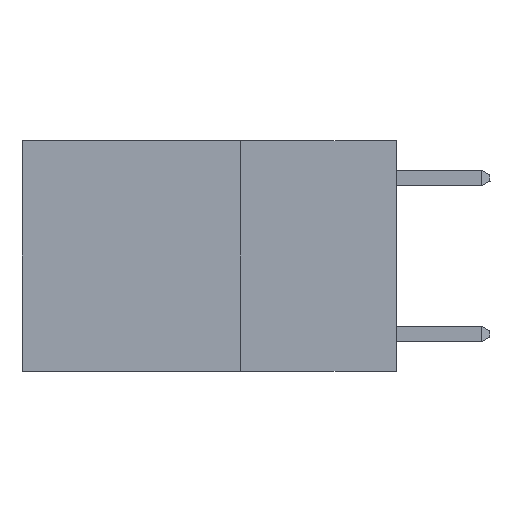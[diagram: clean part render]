
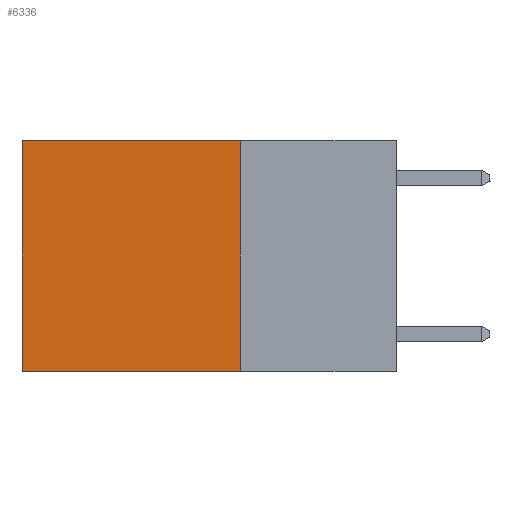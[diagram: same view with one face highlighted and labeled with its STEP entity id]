
A CAD part, left-side view. The second image highlights one B-rep face of the part: STEP entity #6336.
In plain terms, the highlighted planar face has unit normal (-1, 0, 0).
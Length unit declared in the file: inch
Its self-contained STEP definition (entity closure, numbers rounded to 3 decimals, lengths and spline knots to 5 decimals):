
#197 = PLANE ( 'NONE',  #7676 ) ;
#583 = CARTESIAN_POINT ( 'NONE',  ( 0.2625, 0.25, 0. ) ) ;
#915 = EDGE_LOOP ( 'NONE', ( #24273, #24753, #13800, #18570 ) ) ;
#1451 = DIRECTION ( 'NONE',  ( 0., 1., 0. ) ) ;
#1945 = CARTESIAN_POINT ( 'NONE',  ( 0.2625, 0.6, 0. ) ) ;
#2980 = VECTOR ( 'NONE', #15798, 39.37008 ) ;
#5169 = VERTEX_POINT ( 'NONE', #24389 ) ;
#6336 = ADVANCED_FACE ( 'NONE', ( #20495 ), #197, .F. ) ;
#7676 = AXIS2_PLACEMENT_3D ( 'NONE', #17602, #21584, #9922 ) ;
#8330 = CARTESIAN_POINT ( 'NONE',  ( 0.2625, 0.25, 0. ) ) ;
#8669 = LINE ( 'NONE', #9377, #13223 ) ;
#9112 = CARTESIAN_POINT ( 'NONE',  ( 0.2625, 0.25, -0.37 ) ) ;
#9158 = LINE ( 'NONE', #8330, #2980 ) ;
#9377 = CARTESIAN_POINT ( 'NONE',  ( 0.2625, 0.6, 0. ) ) ;
#9922 = DIRECTION ( 'NONE',  ( 0., 0., -1. ) ) ;
#12795 = EDGE_CURVE ( 'NONE', #5169, #16955, #9158, .T. ) ;
#13212 = CARTESIAN_POINT ( 'NONE',  ( 0.2625, 0.25, -0.37 ) ) ;
#13223 = VECTOR ( 'NONE', #19246, 39.37008 ) ;
#13241 = VERTEX_POINT ( 'NONE', #19505 ) ;
#13800 = ORIENTED_EDGE ( 'NONE', *, *, #21367, .F. ) ;
#15798 = DIRECTION ( 'NONE',  ( 0., 1., 0. ) ) ;
#16955 = VERTEX_POINT ( 'NONE', #1945 ) ;
#17602 = CARTESIAN_POINT ( 'NONE',  ( 0.2625, 0.25, 0. ) ) ;
#18570 = ORIENTED_EDGE ( 'NONE', *, *, #12795, .T. ) ;
#19246 = DIRECTION ( 'NONE',  ( 0., 0., -1. ) ) ;
#19505 = CARTESIAN_POINT ( 'NONE',  ( 0.2625, 0.6, -0.37 ) ) ;
#19908 = DIRECTION ( 'NONE',  ( 0., 0., -1. ) ) ;
#20495 = FACE_OUTER_BOUND ( 'NONE', #915, .T. ) ;
#21367 = EDGE_CURVE ( 'NONE', #5169, #21636, #23068, .T. ) ;
#21584 = DIRECTION ( 'NONE',  ( 1., 0., 0. ) ) ;
#21636 = VERTEX_POINT ( 'NONE', #9112 ) ;
#21714 = LINE ( 'NONE', #13212, #23294 ) ;
#22460 = VECTOR ( 'NONE', #19908, 39.37008 ) ;
#22864 = EDGE_CURVE ( 'NONE', #16955, #13241, #8669, .T. ) ;
#22988 = EDGE_CURVE ( 'NONE', #21636, #13241, #21714, .T. ) ;
#23068 = LINE ( 'NONE', #583, #22460 ) ;
#23294 = VECTOR ( 'NONE', #1451, 39.37008 ) ;
#24273 = ORIENTED_EDGE ( 'NONE', *, *, #22864, .T. ) ;
#24389 = CARTESIAN_POINT ( 'NONE',  ( 0.2625, 0.25, 0. ) ) ;
#24753 = ORIENTED_EDGE ( 'NONE', *, *, #22988, .F. ) ;
